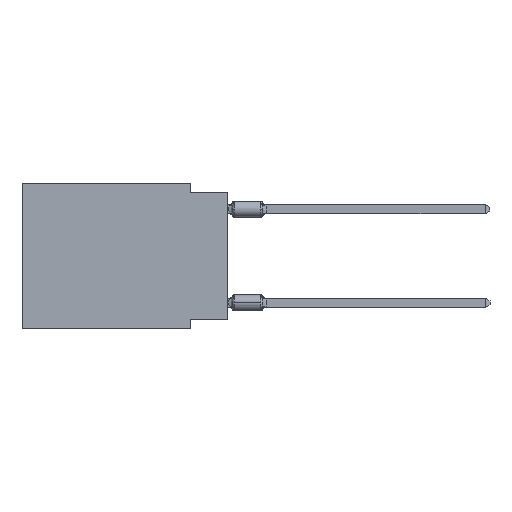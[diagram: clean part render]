
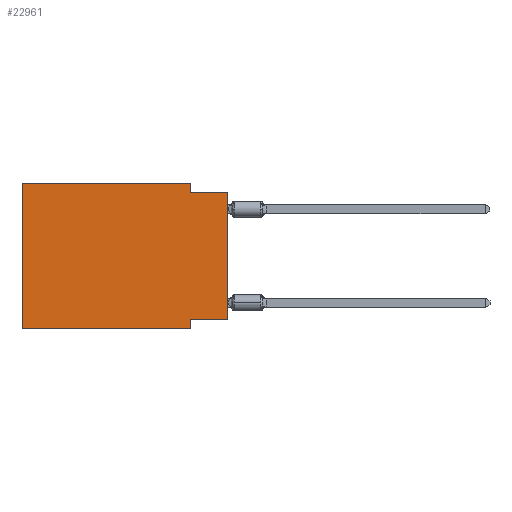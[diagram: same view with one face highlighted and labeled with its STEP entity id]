
A CAD part, left-side view. The second image highlights one B-rep face of the part: STEP entity #22961.
In plain terms, the highlighted planar face has unit normal (-1, 0, 0).
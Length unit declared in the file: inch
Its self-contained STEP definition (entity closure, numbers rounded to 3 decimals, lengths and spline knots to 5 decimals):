
#303 = CARTESIAN_POINT ( 'NONE',  ( 0., 0.55, -0.39 ) ) ;
#392 = AXIS2_PLACEMENT_3D ( 'NONE', #21436, #16901, #16649 ) ;
#898 = DIRECTION ( 'NONE',  ( 0., -1., 0. ) ) ;
#1467 = VERTEX_POINT ( 'NONE', #16945 ) ;
#1763 = EDGE_CURVE ( 'NONE', #25387, #22304, #20969, .T. ) ;
#2177 = LINE ( 'NONE', #14854, #4284 ) ;
#2433 = DIRECTION ( 'NONE',  ( 0., 0., 1. ) ) ;
#3420 = CARTESIAN_POINT ( 'NONE',  ( 0., 0., -0.365 ) ) ;
#4284 = VECTOR ( 'NONE', #10503, 39.37008 ) ;
#4427 = LINE ( 'NONE', #303, #7451 ) ;
#4937 = ORIENTED_EDGE ( 'NONE', *, *, #15972, .T. ) ;
#5557 = CARTESIAN_POINT ( 'NONE',  ( 0., 0.1, -0.39 ) ) ;
#5775 = ORIENTED_EDGE ( 'NONE', *, *, #8966, .F. ) ;
#6471 = VERTEX_POINT ( 'NONE', #24056 ) ;
#7267 = ORIENTED_EDGE ( 'NONE', *, *, #16162, .F. ) ;
#7451 = VECTOR ( 'NONE', #12892, 39.37008 ) ;
#7596 = EDGE_CURVE ( 'NONE', #15930, #23394, #23136, .T. ) ;
#7614 = DIRECTION ( 'NONE',  ( 0., 0., -1. ) ) ;
#7684 = ORIENTED_EDGE ( 'NONE', *, *, #7596, .F. ) ;
#7766 = VECTOR ( 'NONE', #898, 39.37008 ) ;
#7911 = DIRECTION ( 'NONE',  ( 0., 1., 0. ) ) ;
#8225 = VERTEX_POINT ( 'NONE', #18677 ) ;
#8966 = EDGE_CURVE ( 'NONE', #23394, #22447, #23819, .T. ) ;
#10237 = LINE ( 'NONE', #3420, #19570 ) ;
#10351 = CARTESIAN_POINT ( 'NONE',  ( 0., 0.1, 0. ) ) ;
#10356 = FACE_OUTER_BOUND ( 'NONE', #11519, .T. ) ;
#10503 = DIRECTION ( 'NONE',  ( 0., 0., 1. ) ) ;
#10674 = VECTOR ( 'NONE', #23391, 39.37008 ) ;
#11323 = ORIENTED_EDGE ( 'NONE', *, *, #18601, .F. ) ;
#11519 = EDGE_LOOP ( 'NONE', ( #4937, #5775, #7684, #15553, #12283, #23036, #7267, #11323 ) ) ;
#11939 = CARTESIAN_POINT ( 'NONE',  ( 0., 0., -0.025 ) ) ;
#12004 = LINE ( 'NONE', #5557, #13471 ) ;
#12283 = ORIENTED_EDGE ( 'NONE', *, *, #1763, .F. ) ;
#12340 = CARTESIAN_POINT ( 'NONE',  ( 0., 0.55, 0. ) ) ;
#12405 = CARTESIAN_POINT ( 'NONE',  ( 0., 0.55, 0. ) ) ;
#12834 = PLANE ( 'NONE',  #392 ) ;
#12892 = DIRECTION ( 'NONE',  ( 0., -1., 0. ) ) ;
#13471 = VECTOR ( 'NONE', #7614, 39.37008 ) ;
#14657 = CARTESIAN_POINT ( 'NONE',  ( 0., 0.1, -0.025 ) ) ;
#14854 = CARTESIAN_POINT ( 'NONE',  ( 0., 0., 0. ) ) ;
#15553 = ORIENTED_EDGE ( 'NONE', *, *, #25601, .F. ) ;
#15714 = CARTESIAN_POINT ( 'NONE',  ( 0., 0.55, -0.39 ) ) ;
#15930 = VERTEX_POINT ( 'NONE', #10351 ) ;
#15972 = EDGE_CURVE ( 'NONE', #1467, #22447, #2177, .T. ) ;
#16162 = EDGE_CURVE ( 'NONE', #6471, #8225, #12004, .T. ) ;
#16649 = DIRECTION ( 'NONE',  ( 0., 0., -1. ) ) ;
#16901 = DIRECTION ( 'NONE',  ( 1., 0., 0. ) ) ;
#16945 = CARTESIAN_POINT ( 'NONE',  ( 0., 0., -0.365 ) ) ;
#17474 = VECTOR ( 'NONE', #22405, 39.37008 ) ;
#18318 = LINE ( 'NONE', #12340, #17474 ) ;
#18601 = EDGE_CURVE ( 'NONE', #1467, #6471, #10237, .T. ) ;
#18677 = CARTESIAN_POINT ( 'NONE',  ( 0., 0.1, -0.39 ) ) ;
#19570 = VECTOR ( 'NONE', #7911, 39.37008 ) ;
#20670 = EDGE_CURVE ( 'NONE', #25387, #8225, #4427, .T. ) ;
#20969 = LINE ( 'NONE', #12405, #21793 ) ;
#21436 = CARTESIAN_POINT ( 'NONE',  ( 0., 0.55, 0. ) ) ;
#21589 = CARTESIAN_POINT ( 'NONE',  ( 0., 0.55, 0. ) ) ;
#21793 = VECTOR ( 'NONE', #2433, 39.37008 ) ;
#22304 = VERTEX_POINT ( 'NONE', #21589 ) ;
#22405 = DIRECTION ( 'NONE',  ( 0., -1., 0. ) ) ;
#22447 = VERTEX_POINT ( 'NONE', #11939 ) ;
#22961 = ADVANCED_FACE ( 'NONE', ( #10356 ), #12834, .F. ) ;
#23036 = ORIENTED_EDGE ( 'NONE', *, *, #20670, .T. ) ;
#23136 = LINE ( 'NONE', #25047, #10674 ) ;
#23391 = DIRECTION ( 'NONE',  ( 0., 0., -1. ) ) ;
#23394 = VERTEX_POINT ( 'NONE', #14657 ) ;
#23819 = LINE ( 'NONE', #23957, #7766 ) ;
#23957 = CARTESIAN_POINT ( 'NONE',  ( 0., 0., -0.025 ) ) ;
#24056 = CARTESIAN_POINT ( 'NONE',  ( 0., 0.1, -0.365 ) ) ;
#25047 = CARTESIAN_POINT ( 'NONE',  ( 0., 0.1, 0. ) ) ;
#25387 = VERTEX_POINT ( 'NONE', #15714 ) ;
#25601 = EDGE_CURVE ( 'NONE', #22304, #15930, #18318, .T. ) ;
